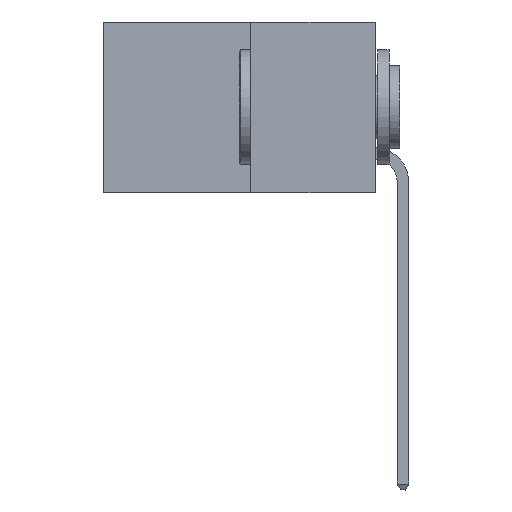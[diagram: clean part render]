
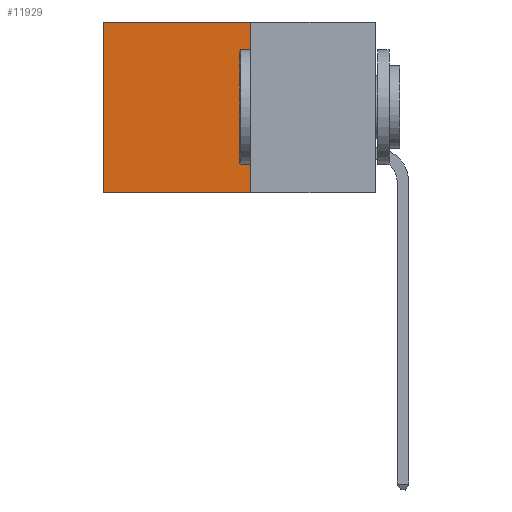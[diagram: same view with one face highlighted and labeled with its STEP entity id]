
A CAD part, left-side view. The second image highlights one B-rep face of the part: STEP entity #11929.
In plain terms, the highlighted planar face has unit normal (-1, 0, 0).
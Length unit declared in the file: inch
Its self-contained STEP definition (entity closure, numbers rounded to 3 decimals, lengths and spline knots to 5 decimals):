
#861 = VECTOR ( 'NONE', #17067, 39.37008 ) ;
#901 = PLANE ( 'NONE',  #17299 ) ;
#1186 = ORIENTED_EDGE ( 'NONE', *, *, #10181, .T. ) ;
#1502 = VECTOR ( 'NONE', #3979, 39.37008 ) ;
#1957 = CARTESIAN_POINT ( 'NONE',  ( 0.277, 0.27, 0. ) ) ;
#1989 = CARTESIAN_POINT ( 'NONE',  ( 0.277, 0.27, -0.37 ) ) ;
#2186 = EDGE_CURVE ( 'NONE', #13084, #6283, #2637, .T. ) ;
#2637 = LINE ( 'NONE', #10404, #6200 ) ;
#3862 = VERTEX_POINT ( 'NONE', #11689 ) ;
#3979 = DIRECTION ( 'NONE',  ( 0., 0., -1. ) ) ;
#5524 = DIRECTION ( 'NONE',  ( 1., 0., 0. ) ) ;
#5562 = LINE ( 'NONE', #14601, #1502 ) ;
#5870 = VERTEX_POINT ( 'NONE', #14275 ) ;
#6200 = VECTOR ( 'NONE', #6704, 39.37008 ) ;
#6283 = VERTEX_POINT ( 'NONE', #12168 ) ;
#6704 = DIRECTION ( 'NONE',  ( 0., 1., 0. ) ) ;
#7232 = DIRECTION ( 'NONE',  ( 0., 0., -1. ) ) ;
#7508 = ORIENTED_EDGE ( 'NONE', *, *, #2186, .T. ) ;
#8780 = VECTOR ( 'NONE', #7232, 39.37008 ) ;
#8785 = CARTESIAN_POINT ( 'NONE',  ( 0.277, 0.27, -0.37 ) ) ;
#9260 = LINE ( 'NONE', #8785, #8780 ) ;
#10029 = FACE_OUTER_BOUND ( 'NONE', #15772, .T. ) ;
#10181 = EDGE_CURVE ( 'NONE', #6283, #5870, #5562, .T. ) ;
#10404 = CARTESIAN_POINT ( 'NONE',  ( 0.277, 0.27, 0. ) ) ;
#11689 = CARTESIAN_POINT ( 'NONE',  ( 0.277, 0.27, -0.37 ) ) ;
#11929 = ADVANCED_FACE ( 'NONE', ( #10029 ), #901, .F. ) ;
#12168 = CARTESIAN_POINT ( 'NONE',  ( 0.277, 0.59, 0. ) ) ;
#13064 = LINE ( 'NONE', #1989, #861 ) ;
#13084 = VERTEX_POINT ( 'NONE', #1957 ) ;
#13728 = ORIENTED_EDGE ( 'NONE', *, *, #18857, .F. ) ;
#13763 = EDGE_CURVE ( 'NONE', #3862, #5870, #13064, .T. ) ;
#14275 = CARTESIAN_POINT ( 'NONE',  ( 0.277, 0.59, -0.37 ) ) ;
#14599 = ORIENTED_EDGE ( 'NONE', *, *, #13763, .F. ) ;
#14601 = CARTESIAN_POINT ( 'NONE',  ( 0.277, 0.59, -0.37 ) ) ;
#14618 = CARTESIAN_POINT ( 'NONE',  ( 0.277, 0.27, -0.37 ) ) ;
#15772 = EDGE_LOOP ( 'NONE', ( #1186, #14599, #13728, #7508 ) ) ;
#16090 = DIRECTION ( 'NONE',  ( 0., 0., -1. ) ) ;
#17067 = DIRECTION ( 'NONE',  ( 0., 1., 0. ) ) ;
#17299 = AXIS2_PLACEMENT_3D ( 'NONE', #14618, #5524, #16090 ) ;
#18857 = EDGE_CURVE ( 'NONE', #13084, #3862, #9260, .T. ) ;
